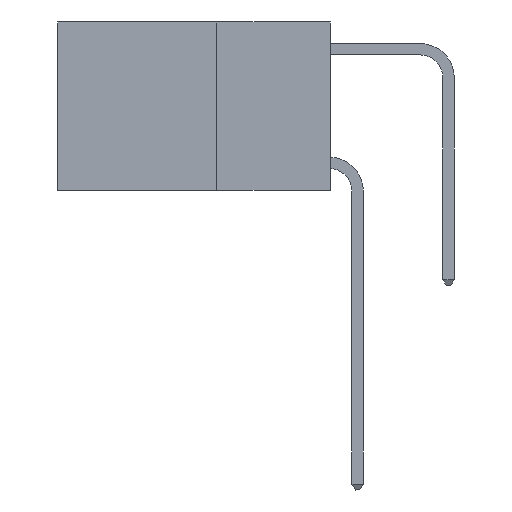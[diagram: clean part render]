
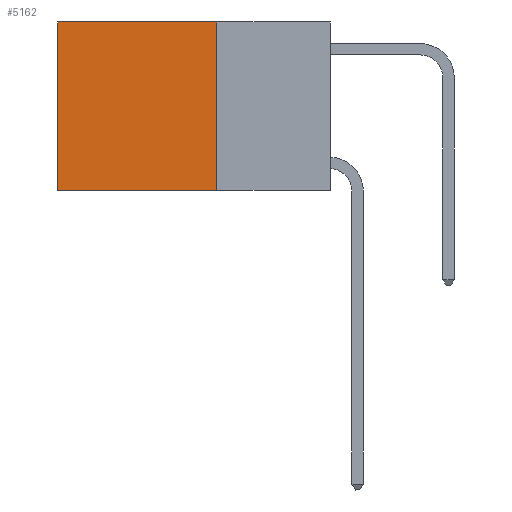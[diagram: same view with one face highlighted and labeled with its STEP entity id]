
A CAD part, left-side view. The second image highlights one B-rep face of the part: STEP entity #5162.
In plain terms, the highlighted planar face has unit normal (-1, 0, 0).
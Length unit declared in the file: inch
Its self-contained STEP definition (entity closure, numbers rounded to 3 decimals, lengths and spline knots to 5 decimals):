
#504 = CARTESIAN_POINT ( 'NONE',  ( 0.2625, 0.25, 0. ) ) ;
#732 = PLANE ( 'NONE',  #10044 ) ;
#769 = DIRECTION ( 'NONE',  ( 0., 0., -1. ) ) ;
#2095 = VECTOR ( 'NONE', #20475, 39.37008 ) ;
#2811 = LINE ( 'NONE', #22494, #2095 ) ;
#3040 = ORIENTED_EDGE ( 'NONE', *, *, #13086, .F. ) ;
#3674 = VERTEX_POINT ( 'NONE', #18049 ) ;
#4415 = CARTESIAN_POINT ( 'NONE',  ( 0.2625, 0.25, 0. ) ) ;
#5162 = ADVANCED_FACE ( 'NONE', ( #9737 ), #732, .F. ) ;
#5291 = CARTESIAN_POINT ( 'NONE',  ( 0.2625, 0.25, 0. ) ) ;
#5393 = ORIENTED_EDGE ( 'NONE', *, *, #8590, .T. ) ;
#5963 = DIRECTION ( 'NONE',  ( 0., 0., -1. ) ) ;
#7311 = VECTOR ( 'NONE', #769, 39.37008 ) ;
#8183 = LINE ( 'NONE', #504, #13987 ) ;
#8384 = EDGE_CURVE ( 'NONE', #3674, #18583, #19759, .T. ) ;
#8590 = EDGE_CURVE ( 'NONE', #18583, #17083, #16999, .T. ) ;
#9064 = DIRECTION ( 'NONE',  ( 0., 1., 0. ) ) ;
#9352 = CARTESIAN_POINT ( 'NONE',  ( 0.2625, 0.6, -0.37 ) ) ;
#9737 = FACE_OUTER_BOUND ( 'NONE', #21767, .T. ) ;
#9845 = DIRECTION ( 'NONE',  ( 0., 0., -1. ) ) ;
#10044 = AXIS2_PLACEMENT_3D ( 'NONE', #4415, #20225, #9845 ) ;
#11552 = CARTESIAN_POINT ( 'NONE',  ( 0.2625, 0.6, 0. ) ) ;
#13086 = EDGE_CURVE ( 'NONE', #21727, #17083, #2811, .T. ) ;
#13987 = VECTOR ( 'NONE', #5963, 39.37008 ) ;
#14583 = CARTESIAN_POINT ( 'NONE',  ( 0.2625, 0.6, 0. ) ) ;
#14892 = CARTESIAN_POINT ( 'NONE',  ( 0.2625, 0.25, -0.37 ) ) ;
#16999 = LINE ( 'NONE', #11552, #7311 ) ;
#17083 = VERTEX_POINT ( 'NONE', #9352 ) ;
#18049 = CARTESIAN_POINT ( 'NONE',  ( 0.2625, 0.25, 0. ) ) ;
#18170 = ORIENTED_EDGE ( 'NONE', *, *, #8384, .T. ) ;
#18583 = VERTEX_POINT ( 'NONE', #14583 ) ;
#18796 = VECTOR ( 'NONE', #9064, 39.37008 ) ;
#19494 = EDGE_CURVE ( 'NONE', #3674, #21727, #8183, .T. ) ;
#19759 = LINE ( 'NONE', #5291, #18796 ) ;
#20225 = DIRECTION ( 'NONE',  ( 1., 0., 0. ) ) ;
#20475 = DIRECTION ( 'NONE',  ( 0., 1., 0. ) ) ;
#21285 = ORIENTED_EDGE ( 'NONE', *, *, #19494, .F. ) ;
#21727 = VERTEX_POINT ( 'NONE', #14892 ) ;
#21767 = EDGE_LOOP ( 'NONE', ( #5393, #3040, #21285, #18170 ) ) ;
#22494 = CARTESIAN_POINT ( 'NONE',  ( 0.2625, 0.25, -0.37 ) ) ;
